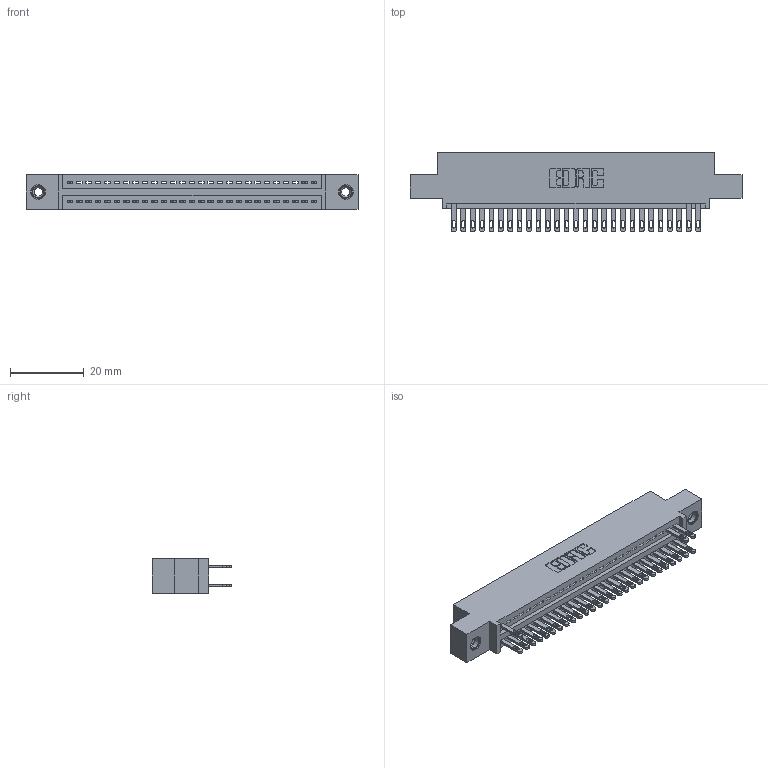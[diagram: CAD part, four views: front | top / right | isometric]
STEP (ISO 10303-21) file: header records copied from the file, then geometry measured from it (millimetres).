
FILE_DESCRIPTION (( 'STEP AP203' ), '1' );
FILE_NAME ('345-054-500-508.STEP', '2018-09-23T19:53:45', ( '' ), ( '' ), 'SwSTEP 2.0', 'SolidWorks 2016', '' );
FILE_SCHEMA (( 'CONFIG_CONTROL_DESIGN' ));
Length unit declared in the file: inch
Products named in the file (4): 345-292-001_345-293-100; 345-250-001_345-250-003-102; 345-054-500-508; 345 Part_0.110 Offset - 0.156 Dia-TI
Assembly tree (33 placements, depth 2):
  345-054-500-508
    345 Part_0.110 Offset - 0.156 Dia-TI
    345-292-001_345-293-100  x30
    345-250-001_345-250-003-102  x2
Bounding box: 89.79 x 21.51 x 9.4 mm (x, y, z)
Volume: 8378.4 mm3; surface area: 11281.1 mm2
Topology: 33 solids, 33 shells, 1762 faces, 5367 edges, 3570 vertices
Faces by surface type: plane 1094, cylinder 652, cone 12, torus 4
Entity records: 23684 total; most frequent: CARTESIAN_POINT 4071, ORIENTED_EDGE 4022, DIRECTION 3609, EDGE_CURVE 2011, VECTOR 1747, LINE 1747, VERTEX_POINT 1336, AXIS2_PLACEMENT_3D 931
